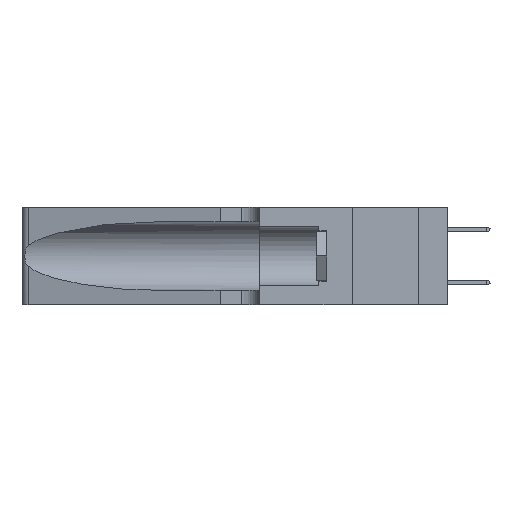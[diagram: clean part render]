
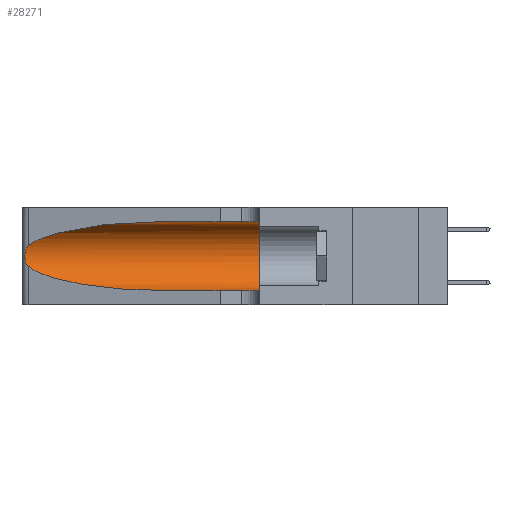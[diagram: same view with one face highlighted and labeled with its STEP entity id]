
A CAD part, left-side view. The second image highlights one B-rep face of the part: STEP entity #28271.
In plain terms, the highlighted cylindrical face has radius 3.308 mm (diameter 6.617 mm), a partial arc.
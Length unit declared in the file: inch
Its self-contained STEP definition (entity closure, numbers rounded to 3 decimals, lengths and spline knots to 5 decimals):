
#430 =( BOUNDED_CURVE ( )  B_SPLINE_CURVE ( 3, ( #20554, #27336, #2084, #38305 ),
 .UNSPECIFIED., .F., .T. ) 
 B_SPLINE_CURVE_WITH_KNOTS ( ( 4, 4 ),
 ( 1.5708, 2.84003 ),
 .UNSPECIFIED. ) 
 CURVE ( )  GEOMETRIC_REPRESENTATION_ITEM ( )  RATIONAL_B_SPLINE_CURVE ( ( 1., 0.87, 0.87, 1. ) ) 
 REPRESENTATION_ITEM ( '' )  );
#535 = CARTESIAN_POINT ( 'NONE',  ( 0.25487, 1.22718, 0.14631 ) ) ;
#850 = VERTEX_POINT ( 'NONE', #29639 ) ;
#1399 = DIRECTION ( 'NONE',  ( 0., -1., 0. ) ) ;
#2084 = CARTESIAN_POINT ( 'NONE',  ( 0.2373, 1.15595, 0.28018 ) ) ;
#2840 = CARTESIAN_POINT ( 'NONE',  ( 0.1305, 1.61858, 0.05475 ) ) ;
#3002 = DIRECTION ( 'NONE',  ( 0., -1., 0. ) ) ;
#3507 = CARTESIAN_POINT ( 'NONE',  ( 0.25639, 1.23184, 0.21858 ) ) ;
#4459 = CARTESIAN_POINT ( 'NONE',  ( 0.26018, 1.23835, 0.19895 ) ) ;
#4949 = CARTESIAN_POINT ( 'NONE',  ( 0.2373, 1.15595, 0.08982 ) ) ;
#5405 =( BOUNDED_CURVE ( )  B_SPLINE_CURVE ( 3, ( #8758, #4949, #12121, #34159 ),
 .UNSPECIFIED., .F., .F. ) 
 B_SPLINE_CURVE_WITH_KNOTS ( ( 4, 4 ),
 ( 3.44316, 4.71239 ),
 .UNSPECIFIED. ) 
 CURVE ( )  GEOMETRIC_REPRESENTATION_ITEM ( )  RATIONAL_B_SPLINE_CURVE ( ( 1., 0.87, 0.87, 1. ) ) 
 REPRESENTATION_ITEM ( '' )  );
#7200 = VERTEX_POINT ( 'NONE', #19099 ) ;
#8033 = CARTESIAN_POINT ( 'NONE',  ( 0.25487, 1.22718, 0.22369 ) ) ;
#8120 = CARTESIAN_POINT ( 'NONE',  ( 0.25487, 1.22718, 0.14631 ) ) ;
#8270 = CARTESIAN_POINT ( 'NONE',  ( 0.25789, 1.23486, 0.15765 ) ) ;
#8758 = CARTESIAN_POINT ( 'NONE',  ( 0.25487, 1.22718, 0.14631 ) ) ;
#10817 = CARTESIAN_POINT ( 'NONE',  ( 0.25555, 1.22993, 0.14849 ) ) ;
#11094 = EDGE_CURVE ( 'NONE', #7200, #40493, #14677, .T. ) ;
#11434 = VERTEX_POINT ( 'NONE', #27492 ) ;
#12121 = CARTESIAN_POINT ( 'NONE',  ( 0.18966, 0.96281, 0.05475 ) ) ;
#14677 = CIRCLE ( 'NONE', #19687, 0.13025 ) ;
#14892 = LINE ( 'NONE', #44445, #38133 ) ;
#15297 = CARTESIAN_POINT ( 'NONE',  ( 0.25787, 1.23484, 0.2124 ) ) ;
#15414 = CYLINDRICAL_SURFACE ( 'NONE', #41363, 0.13025 ) ;
#15612 = CARTESIAN_POINT ( 'NONE',  ( 0.25639, 1.23186, 0.15144 ) ) ;
#15814 = DIRECTION ( 'NONE',  ( 0., -1., 0. ) ) ;
#16041 = ORIENTED_EDGE ( 'NONE', *, *, #37770, .T. ) ;
#18215 = FACE_OUTER_BOUND ( 'NONE', #23442, .T. ) ;
#19099 = CARTESIAN_POINT ( 'NONE',  ( 0.1305, 0.35, 0.31525 ) ) ;
#19352 = ORIENTED_EDGE ( 'NONE', *, *, #44355, .F. ) ;
#19687 = AXIS2_PLACEMENT_3D ( 'NONE', #26749, #33912, #29909 ) ;
#20554 = CARTESIAN_POINT ( 'NONE',  ( 0.1305, 0.72297, 0.31525 ) ) ;
#21916 = EDGE_CURVE ( 'NONE', #11434, #40493, #22623, .T. ) ;
#22569 = CARTESIAN_POINT ( 'NONE',  ( 0.25854, 1.2359, 0.20912 ) ) ;
#22623 = LINE ( 'NONE', #2840, #27672 ) ;
#22755 = ORIENTED_EDGE ( 'NONE', *, *, #45689, .T. ) ;
#23442 = EDGE_LOOP ( 'NONE', ( #22755, #36068, #16041, #31233, #35722, #19352 ) ) ;
#23701 = CARTESIAN_POINT ( 'NONE',  ( 0.1305, 1.61858, 0.185 ) ) ;
#25238 = CARTESIAN_POINT ( 'NONE',  ( 0.25555, 1.22994, 0.2215 ) ) ;
#26749 = CARTESIAN_POINT ( 'NONE',  ( 0.1305, 0.35, 0.185 ) ) ;
#27336 = CARTESIAN_POINT ( 'NONE',  ( 0.18966, 0.96281, 0.31525 ) ) ;
#27492 = CARTESIAN_POINT ( 'NONE',  ( 0.1305, 0.72297, 0.05475 ) ) ;
#27672 = VECTOR ( 'NONE', #3002, 39.37008 ) ;
#28271 = ADVANCED_FACE ( 'NONE', ( #18215 ), #15414, .F. ) ;
#28740 = EDGE_CURVE ( 'NONE', #38904, #32370, #44085, .T. ) ;
#28880 = CARTESIAN_POINT ( 'NONE',  ( 0.26075, 1.23896, 0.19203 ) ) ;
#29639 = CARTESIAN_POINT ( 'NONE',  ( 0.1305, 0.72297, 0.31525 ) ) ;
#29834 = CARTESIAN_POINT ( 'NONE',  ( 0.26075, 1.23896, 0.178 ) ) ;
#29909 = DIRECTION ( 'NONE',  ( 0., 0., 1. ) ) ;
#31233 = ORIENTED_EDGE ( 'NONE', *, *, #21916, .T. ) ;
#32370 = VERTEX_POINT ( 'NONE', #535 ) ;
#33912 = DIRECTION ( 'NONE',  ( 0., 1., 0. ) ) ;
#34159 = CARTESIAN_POINT ( 'NONE',  ( 0.1305, 0.72297, 0.05475 ) ) ;
#35722 = ORIENTED_EDGE ( 'NONE', *, *, #11094, .F. ) ;
#36068 = ORIENTED_EDGE ( 'NONE', *, *, #28740, .T. ) ;
#37312 = CARTESIAN_POINT ( 'NONE',  ( 0.26017, 1.23833, 0.17102 ) ) ;
#37770 = EDGE_CURVE ( 'NONE', #32370, #11434, #5405, .T. ) ;
#38133 = VECTOR ( 'NONE', #1399, 39.37008 ) ;
#38305 = CARTESIAN_POINT ( 'NONE',  ( 0.25487, 1.22718, 0.22369 ) ) ;
#38904 = VERTEX_POINT ( 'NONE', #8033 ) ;
#40493 = VERTEX_POINT ( 'NONE', #41798 ) ;
#41363 = AXIS2_PLACEMENT_3D ( 'NONE', #23701, #15814, #45263 ) ;
#41798 = CARTESIAN_POINT ( 'NONE',  ( 0.1305, 0.35, 0.05475 ) ) ;
#44085 = B_SPLINE_CURVE_WITH_KNOTS ( 'NONE', 3,
 ( #44291, #25238, #3507, #15297, #22569, #4459, #28880, #29834, #37312, #44601, #8270, #15612, #10817, #8120 ),
 .UNSPECIFIED., .F., .F.,
 ( 4, 2, 2, 2, 2, 2, 4 ),
 ( 0., 0.00027, 0.00053, 0.00107, 0.0016, 0.00187, 0.00214 ),
 .UNSPECIFIED. ) ;
#44291 = CARTESIAN_POINT ( 'NONE',  ( 0.25487, 1.22718, 0.22369 ) ) ;
#44355 = EDGE_CURVE ( 'NONE', #850, #7200, #14892, .T. ) ;
#44445 = CARTESIAN_POINT ( 'NONE',  ( 0.1305, 1.61858, 0.31525 ) ) ;
#44601 = CARTESIAN_POINT ( 'NONE',  ( 0.25856, 1.23593, 0.16098 ) ) ;
#45263 = DIRECTION ( 'NONE',  ( 0., 0., -1. ) ) ;
#45689 = EDGE_CURVE ( 'NONE', #850, #38904, #430, .T. ) ;
